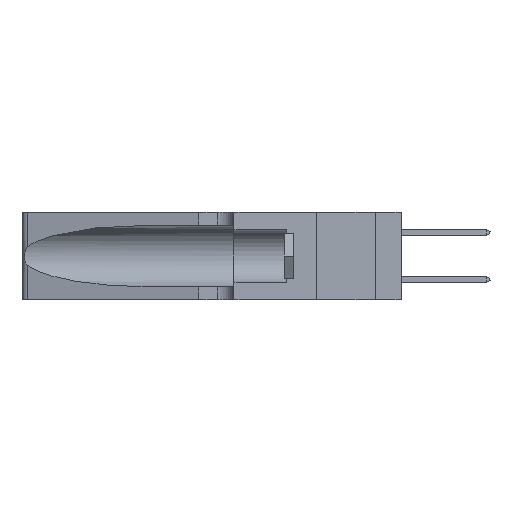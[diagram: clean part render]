
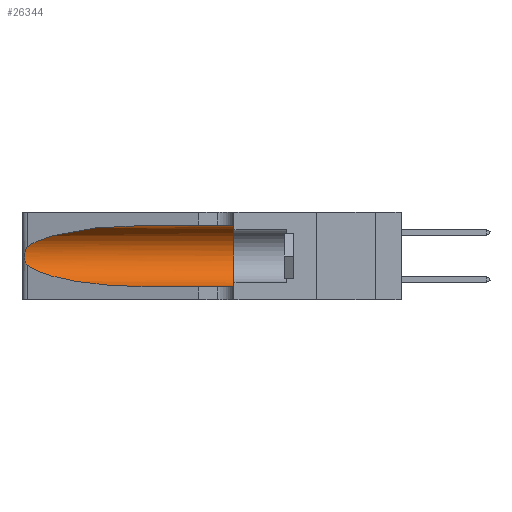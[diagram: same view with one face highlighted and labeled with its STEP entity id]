
A CAD part, left-side view. The second image highlights one B-rep face of the part: STEP entity #26344.
In plain terms, the highlighted cylindrical face has radius 3.308 mm (diameter 6.617 mm), a partial arc.
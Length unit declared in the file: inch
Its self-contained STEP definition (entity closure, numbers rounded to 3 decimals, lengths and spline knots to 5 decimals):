
#80 = ORIENTED_EDGE ( 'NONE', *, *, #7809, .T. ) ;
#565 = CARTESIAN_POINT ( 'NONE',  ( 0.18966, 0.96281, 0.05475 ) ) ;
#1102 = VERTEX_POINT ( 'NONE', #18915 ) ;
#1636 = EDGE_LOOP ( 'NONE', ( #80, #28909, #5240, #6995, #22161, #3880 ) ) ;
#1651 = DIRECTION ( 'NONE',  ( 0., -1., 0. ) ) ;
#2432 = CARTESIAN_POINT ( 'NONE',  ( 0.26075, 1.23896, 0.178 ) ) ;
#3544 = AXIS2_PLACEMENT_3D ( 'NONE', #19648, #4162, #22223 ) ;
#3880 = ORIENTED_EDGE ( 'NONE', *, *, #12969, .F. ) ;
#4155 = DIRECTION ( 'NONE',  ( 0., -1., 0. ) ) ;
#4162 = DIRECTION ( 'NONE',  ( 0., 1., 0. ) ) ;
#4347 = FACE_OUTER_BOUND ( 'NONE', #1636, .T. ) ;
#4518 = CARTESIAN_POINT ( 'NONE',  ( 0.1305, 0.72297, 0.05475 ) ) ;
#4692 = EDGE_CURVE ( 'NONE', #1102, #16378, #19171, .T. ) ;
#4872 = EDGE_CURVE ( 'NONE', #16378, #10463, #13234, .T. ) ;
#5047 = CARTESIAN_POINT ( 'NONE',  ( 0.25856, 1.23593, 0.16098 ) ) ;
#5240 = ORIENTED_EDGE ( 'NONE', *, *, #4872, .T. ) ;
#6427 = CIRCLE ( 'NONE', #3544, 0.13025 ) ;
#6499 = EDGE_CURVE ( 'NONE', #27679, #29105, #6427, .T. ) ;
#6995 = ORIENTED_EDGE ( 'NONE', *, *, #12421, .T. ) ;
#7172 =( BOUNDED_CURVE ( )  B_SPLINE_CURVE ( 3, ( #22974, #25508, #10233, #28076 ),
 .UNSPECIFIED., .F., .F. ) 
 B_SPLINE_CURVE_WITH_KNOTS ( ( 4, 4 ),
 ( 1.5708, 2.84003 ),
 .UNSPECIFIED. ) 
 CURVE ( )  GEOMETRIC_REPRESENTATION_ITEM ( )  RATIONAL_B_SPLINE_CURVE ( ( 1., 0.87, 0.87, 1. ) ) 
 REPRESENTATION_ITEM ( '' )  );
#7704 = CARTESIAN_POINT ( 'NONE',  ( 0.25639, 1.23186, 0.15144 ) ) ;
#7809 = EDGE_CURVE ( 'NONE', #22349, #1102, #7172, .T. ) ;
#9537 = DIRECTION ( 'NONE',  ( 0., 0., -1. ) ) ;
#10233 = CARTESIAN_POINT ( 'NONE',  ( 0.2373, 1.15595, 0.28018 ) ) ;
#10322 = CARTESIAN_POINT ( 'NONE',  ( 0.25487, 1.22718, 0.14631 ) ) ;
#10463 = VERTEX_POINT ( 'NONE', #4518 ) ;
#12421 = EDGE_CURVE ( 'NONE', #10463, #29105, #29640, .T. ) ;
#12839 = CARTESIAN_POINT ( 'NONE',  ( 0.25639, 1.23184, 0.21858 ) ) ;
#12969 = EDGE_CURVE ( 'NONE', #22349, #27679, #18878, .T. ) ;
#13234 =( BOUNDED_CURVE ( )  B_SPLINE_CURVE ( 3, ( #31418, #28824, #565, #18746 ),
 .UNSPECIFIED., .F., .F. ) 
 B_SPLINE_CURVE_WITH_KNOTS ( ( 4, 4 ),
 ( 3.44316, 4.71239 ),
 .UNSPECIFIED. ) 
 CURVE ( )  GEOMETRIC_REPRESENTATION_ITEM ( )  RATIONAL_B_SPLINE_CURVE ( ( 1., 0.87, 0.87, 1. ) ) 
 REPRESENTATION_ITEM ( '' )  );
#14223 = CARTESIAN_POINT ( 'NONE',  ( 0.25487, 1.22718, 0.14631 ) ) ;
#14790 = AXIS2_PLACEMENT_3D ( 'NONE', #24843, #1651, #9537 ) ;
#15319 = VECTOR ( 'NONE', #17453, 39.37008 ) ;
#15411 = CARTESIAN_POINT ( 'NONE',  ( 0.25854, 1.2359, 0.20912 ) ) ;
#16378 = VERTEX_POINT ( 'NONE', #14223 ) ;
#17332 = CYLINDRICAL_SURFACE ( 'NONE', #14790, 0.13025 ) ;
#17453 = DIRECTION ( 'NONE',  ( 0., -1., 0. ) ) ;
#17979 = CARTESIAN_POINT ( 'NONE',  ( 0.26075, 1.23896, 0.19203 ) ) ;
#18075 = VECTOR ( 'NONE', #4155, 39.37008 ) ;
#18746 = CARTESIAN_POINT ( 'NONE',  ( 0.1305, 0.72297, 0.05475 ) ) ;
#18878 = LINE ( 'NONE', #27062, #18075 ) ;
#18915 = CARTESIAN_POINT ( 'NONE',  ( 0.25487, 1.22718, 0.22369 ) ) ;
#19171 = B_SPLINE_CURVE_WITH_KNOTS ( 'NONE', 3,
 ( #25482, #28051, #12839, #30634, #15411, #33192, #17979, #2432, #20522, #5047, #23067, #7704, #25596, #10322 ),
 .UNSPECIFIED., .F., .F.,
 ( 4, 2, 2, 2, 2, 2, 4 ),
 ( 0., 0.00027, 0.00053, 0.00107, 0.0016, 0.00187, 0.00214 ),
 .UNSPECIFIED. ) ;
#19648 = CARTESIAN_POINT ( 'NONE',  ( 0.1305, 0.35, 0.185 ) ) ;
#20522 = CARTESIAN_POINT ( 'NONE',  ( 0.26017, 1.23833, 0.17102 ) ) ;
#22161 = ORIENTED_EDGE ( 'NONE', *, *, #6499, .F. ) ;
#22223 = DIRECTION ( 'NONE',  ( 0., 0., 1. ) ) ;
#22349 = VERTEX_POINT ( 'NONE', #32083 ) ;
#22562 = CARTESIAN_POINT ( 'NONE',  ( 0.1305, 1.61858, 0.05475 ) ) ;
#22974 = CARTESIAN_POINT ( 'NONE',  ( 0.1305, 0.72297, 0.31525 ) ) ;
#23067 = CARTESIAN_POINT ( 'NONE',  ( 0.25789, 1.23486, 0.15765 ) ) ;
#24843 = CARTESIAN_POINT ( 'NONE',  ( 0.1305, 1.61858, 0.185 ) ) ;
#25482 = CARTESIAN_POINT ( 'NONE',  ( 0.25487, 1.22718, 0.22369 ) ) ;
#25508 = CARTESIAN_POINT ( 'NONE',  ( 0.18966, 0.96281, 0.31525 ) ) ;
#25596 = CARTESIAN_POINT ( 'NONE',  ( 0.25555, 1.22993, 0.14849 ) ) ;
#26344 = ADVANCED_FACE ( 'NONE', ( #4347 ), #17332, .F. ) ;
#27062 = CARTESIAN_POINT ( 'NONE',  ( 0.1305, 1.61858, 0.31525 ) ) ;
#27679 = VERTEX_POINT ( 'NONE', #30145 ) ;
#28051 = CARTESIAN_POINT ( 'NONE',  ( 0.25555, 1.22994, 0.2215 ) ) ;
#28076 = CARTESIAN_POINT ( 'NONE',  ( 0.25487, 1.22718, 0.22369 ) ) ;
#28824 = CARTESIAN_POINT ( 'NONE',  ( 0.2373, 1.15595, 0.08982 ) ) ;
#28909 = ORIENTED_EDGE ( 'NONE', *, *, #4692, .T. ) ;
#29105 = VERTEX_POINT ( 'NONE', #30982 ) ;
#29640 = LINE ( 'NONE', #22562, #15319 ) ;
#30145 = CARTESIAN_POINT ( 'NONE',  ( 0.1305, 0.35, 0.31525 ) ) ;
#30634 = CARTESIAN_POINT ( 'NONE',  ( 0.25787, 1.23484, 0.2124 ) ) ;
#30982 = CARTESIAN_POINT ( 'NONE',  ( 0.1305, 0.35, 0.05475 ) ) ;
#31418 = CARTESIAN_POINT ( 'NONE',  ( 0.25487, 1.22718, 0.14631 ) ) ;
#32083 = CARTESIAN_POINT ( 'NONE',  ( 0.1305, 0.72297, 0.31525 ) ) ;
#33192 = CARTESIAN_POINT ( 'NONE',  ( 0.26018, 1.23835, 0.19895 ) ) ;
